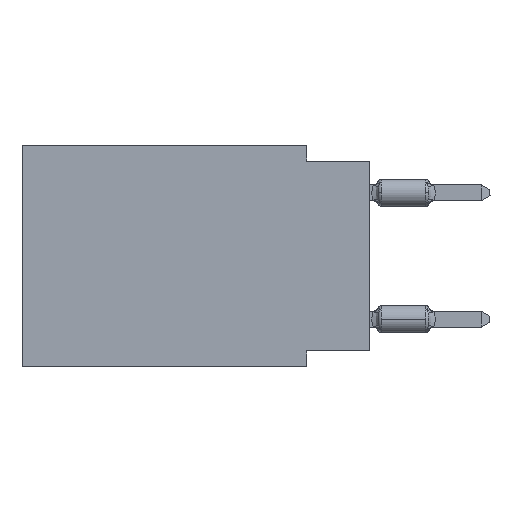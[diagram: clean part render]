
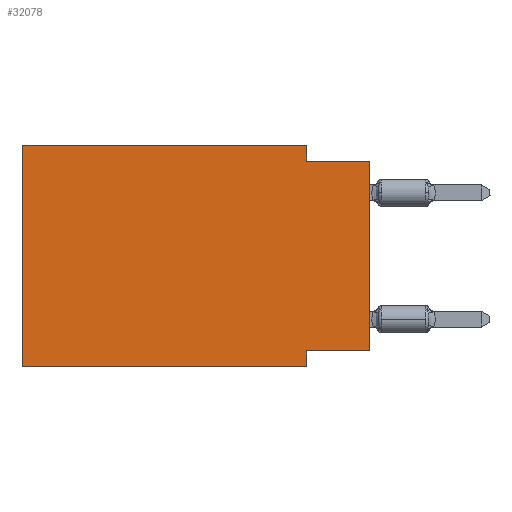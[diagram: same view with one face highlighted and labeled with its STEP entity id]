
A CAD part, left-side view. The second image highlights one B-rep face of the part: STEP entity #32078.
In plain terms, the highlighted planar face has unit normal (-1, 0, 0).
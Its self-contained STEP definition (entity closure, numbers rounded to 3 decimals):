
#130 = EDGE_LOOP ( 'NONE', ( #26047, #30363, #13545, #19799, #19961, #27798, #1799, #33250 ) ) ;
#1799 = ORIENTED_EDGE ( 'NONE', *, *, #18486, .F. ) ;
#5808 = VERTEX_POINT ( 'NONE', #16751 ) ;
#7016 = CARTESIAN_POINT ( 'NONE',  ( 0., 13.97, 0. ) ) ;
#7657 = CARTESIAN_POINT ( 'NONE',  ( 0., 0., -0.635 ) ) ;
#8154 = EDGE_CURVE ( 'NONE', #25112, #42571, #22268, .T. ) ;
#9092 = LINE ( 'NONE', #17144, #17246 ) ;
#9464 = DIRECTION ( 'NONE',  ( 0., 1., 0. ) ) ;
#10744 = VECTOR ( 'NONE', #21353, 1000. ) ;
#10858 = VECTOR ( 'NONE', #41781, 1000. ) ;
#11326 = CARTESIAN_POINT ( 'NONE',  ( 0., 2.54, 0. ) ) ;
#11814 = EDGE_CURVE ( 'NONE', #20878, #5808, #26641, .T. ) ;
#13075 = DIRECTION ( 'NONE',  ( 1., 0., 0. ) ) ;
#13545 = ORIENTED_EDGE ( 'NONE', *, *, #39019, .F. ) ;
#14182 = LINE ( 'NONE', #7657, #10744 ) ;
#14411 = LINE ( 'NONE', #28092, #10858 ) ;
#15027 = CARTESIAN_POINT ( 'NONE',  ( 0., 2.54, -8.89 ) ) ;
#16751 = CARTESIAN_POINT ( 'NONE',  ( 0., 2.54, 0. ) ) ;
#17092 = FACE_OUTER_BOUND ( 'NONE', #130, .T. ) ;
#17144 = CARTESIAN_POINT ( 'NONE',  ( 0., 0., 0. ) ) ;
#17246 = VECTOR ( 'NONE', #37569, 1000. ) ;
#17553 = CARTESIAN_POINT ( 'NONE',  ( 0., 13.97, 0. ) ) ;
#17857 = VERTEX_POINT ( 'NONE', #18435 ) ;
#17931 = EDGE_CURVE ( 'NONE', #17857, #32263, #14411, .T. ) ;
#18435 = CARTESIAN_POINT ( 'NONE',  ( 0., 13.97, -8.89 ) ) ;
#18486 = EDGE_CURVE ( 'NONE', #42571, #32263, #28706, .T. ) ;
#19589 = PLANE ( 'NONE',  #27973 ) ;
#19799 = ORIENTED_EDGE ( 'NONE', *, *, #11814, .F. ) ;
#19961 = ORIENTED_EDGE ( 'NONE', *, *, #25997, .F. ) ;
#20468 = DIRECTION ( 'NONE',  ( 0., 0., 1. ) ) ;
#20878 = VERTEX_POINT ( 'NONE', #17553 ) ;
#21353 = DIRECTION ( 'NONE',  ( 0., -1., 0. ) ) ;
#22268 = LINE ( 'NONE', #30104, #31939 ) ;
#23630 = EDGE_CURVE ( 'NONE', #25112, #34279, #9092, .T. ) ;
#24345 = EDGE_CURVE ( 'NONE', #25712, #34279, #14182, .T. ) ;
#24794 = LINE ( 'NONE', #11326, #43825 ) ;
#25112 = VERTEX_POINT ( 'NONE', #25230 ) ;
#25230 = CARTESIAN_POINT ( 'NONE',  ( 0., 0., -8.255 ) ) ;
#25712 = VERTEX_POINT ( 'NONE', #42729 ) ;
#25997 = EDGE_CURVE ( 'NONE', #17857, #20878, #30581, .T. ) ;
#26047 = ORIENTED_EDGE ( 'NONE', *, *, #23630, .T. ) ;
#26550 = DIRECTION ( 'NONE',  ( 0., 0., -1. ) ) ;
#26641 = LINE ( 'NONE', #37174, #40767 ) ;
#26989 = VECTOR ( 'NONE', #20468, 1000. ) ;
#27798 = ORIENTED_EDGE ( 'NONE', *, *, #17931, .T. ) ;
#27973 = AXIS2_PLACEMENT_3D ( 'NONE', #43617, #13075, #26550 ) ;
#28092 = CARTESIAN_POINT ( 'NONE',  ( 0., 13.97, -8.89 ) ) ;
#28193 = CARTESIAN_POINT ( 'NONE',  ( 0., 2.54, -8.255 ) ) ;
#28706 = LINE ( 'NONE', #15027, #38142 ) ;
#30104 = CARTESIAN_POINT ( 'NONE',  ( 0., 0., -8.255 ) ) ;
#30363 = ORIENTED_EDGE ( 'NONE', *, *, #24345, .F. ) ;
#30581 = LINE ( 'NONE', #7016, #26989 ) ;
#31939 = VECTOR ( 'NONE', #9464, 1000. ) ;
#32078 = ADVANCED_FACE ( 'NONE', ( #17092 ), #19589, .F. ) ;
#32263 = VERTEX_POINT ( 'NONE', #39060 ) ;
#32298 = DIRECTION ( 'NONE',  ( 0., 0., -1. ) ) ;
#33250 = ORIENTED_EDGE ( 'NONE', *, *, #8154, .F. ) ;
#34279 = VERTEX_POINT ( 'NONE', #40605 ) ;
#37174 = CARTESIAN_POINT ( 'NONE',  ( 0., 13.97, 0. ) ) ;
#37569 = DIRECTION ( 'NONE',  ( 0., 0., 1. ) ) ;
#38142 = VECTOR ( 'NONE', #32298, 1000. ) ;
#39019 = EDGE_CURVE ( 'NONE', #5808, #25712, #24794, .T. ) ;
#39060 = CARTESIAN_POINT ( 'NONE',  ( 0., 2.54, -8.89 ) ) ;
#40334 = DIRECTION ( 'NONE',  ( 0., -1., 0. ) ) ;
#40605 = CARTESIAN_POINT ( 'NONE',  ( 0., 0., -0.635 ) ) ;
#40767 = VECTOR ( 'NONE', #40334, 1000. ) ;
#41633 = DIRECTION ( 'NONE',  ( 0., 0., -1. ) ) ;
#41781 = DIRECTION ( 'NONE',  ( 0., -1., 0. ) ) ;
#42571 = VERTEX_POINT ( 'NONE', #28193 ) ;
#42729 = CARTESIAN_POINT ( 'NONE',  ( 0., 2.54, -0.635 ) ) ;
#43617 = CARTESIAN_POINT ( 'NONE',  ( 0., 13.97, 0. ) ) ;
#43825 = VECTOR ( 'NONE', #41633, 1000. ) ;
